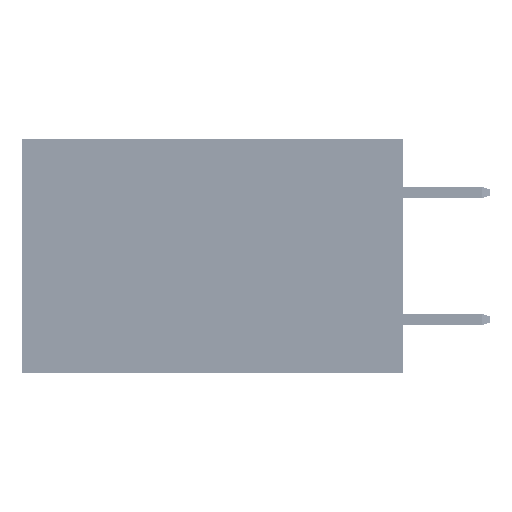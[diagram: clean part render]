
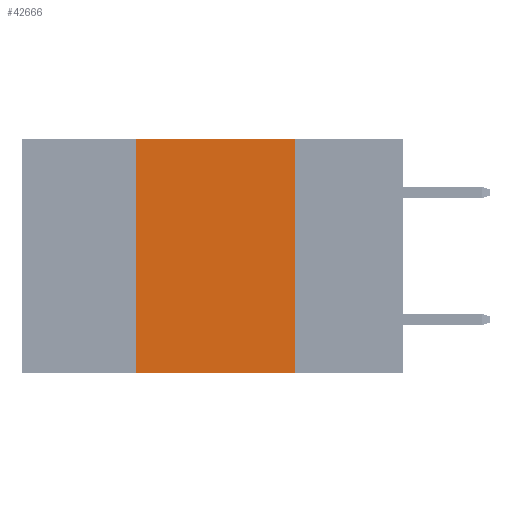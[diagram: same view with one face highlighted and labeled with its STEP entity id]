
A CAD part, left-side view. The second image highlights one B-rep face of the part: STEP entity #42666.
In plain terms, the highlighted planar face has unit normal (-1, 0, 0).
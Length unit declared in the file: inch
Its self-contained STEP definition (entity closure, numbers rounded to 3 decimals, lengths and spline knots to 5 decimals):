
#2341 = DIRECTION ( 'NONE',  ( 1., 0., 0. ) ) ;
#2729 = VERTEX_POINT ( 'NONE', #36102 ) ;
#5283 = CARTESIAN_POINT ( 'NONE',  ( 0., 0.17, -0.37 ) ) ;
#5970 = LINE ( 'NONE', #47476, #14179 ) ;
#6829 = DIRECTION ( 'NONE',  ( 0., -1., 0. ) ) ;
#9076 = DIRECTION ( 'NONE',  ( 0., -1., 0. ) ) ;
#9481 = LINE ( 'NONE', #24145, #21701 ) ;
#11078 = DIRECTION ( 'NONE',  ( 0., 0., 1. ) ) ;
#13001 = CARTESIAN_POINT ( 'NONE',  ( 0., 0.6, 0. ) ) ;
#13865 = VECTOR ( 'NONE', #6829, 39.37008 ) ;
#14179 = VECTOR ( 'NONE', #9076, 39.37008 ) ;
#21701 = VECTOR ( 'NONE', #32241, 39.37008 ) ;
#24145 = CARTESIAN_POINT ( 'NONE',  ( 0., 0.17, 0. ) ) ;
#26279 = CARTESIAN_POINT ( 'NONE',  ( 0., 0.42, 0. ) ) ;
#26647 = EDGE_CURVE ( 'NONE', #44932, #35013, #5970, .T. ) ;
#27323 = VECTOR ( 'NONE', #11078, 39.37008 ) ;
#28458 = PLANE ( 'NONE',  #36567 ) ;
#29786 = VERTEX_POINT ( 'NONE', #30401 ) ;
#30401 = CARTESIAN_POINT ( 'NONE',  ( 0., 0.17, 0. ) ) ;
#32241 = DIRECTION ( 'NONE',  ( 0., 0., -1. ) ) ;
#33123 = LINE ( 'NONE', #26279, #27323 ) ;
#33491 = DIRECTION ( 'NONE',  ( 0., 0., -1. ) ) ;
#34145 = ORIENTED_EDGE ( 'NONE', *, *, #35557, .F. ) ;
#34201 = CARTESIAN_POINT ( 'NONE',  ( 0., 0.6, 0. ) ) ;
#35013 = VERTEX_POINT ( 'NONE', #5283 ) ;
#35150 = EDGE_CURVE ( 'NONE', #2729, #29786, #41501, .T. ) ;
#35557 = EDGE_CURVE ( 'NONE', #44932, #2729, #33123, .T. ) ;
#36102 = CARTESIAN_POINT ( 'NONE',  ( 0., 0.42, 0. ) ) ;
#36290 = FACE_OUTER_BOUND ( 'NONE', #45259, .T. ) ;
#36300 = EDGE_CURVE ( 'NONE', #29786, #35013, #9481, .T. ) ;
#36567 = AXIS2_PLACEMENT_3D ( 'NONE', #13001, #2341, #33491 ) ;
#40978 = ORIENTED_EDGE ( 'NONE', *, *, #35150, .F. ) ;
#41501 = LINE ( 'NONE', #34201, #13865 ) ;
#42666 = ADVANCED_FACE ( 'NONE', ( #36290 ), #28458, .F. ) ;
#44439 = ORIENTED_EDGE ( 'NONE', *, *, #26647, .T. ) ;
#44932 = VERTEX_POINT ( 'NONE', #46752 ) ;
#45259 = EDGE_LOOP ( 'NONE', ( #46855, #40978, #34145, #44439 ) ) ;
#46752 = CARTESIAN_POINT ( 'NONE',  ( 0., 0.42, -0.37 ) ) ;
#46855 = ORIENTED_EDGE ( 'NONE', *, *, #36300, .F. ) ;
#47476 = CARTESIAN_POINT ( 'NONE',  ( 0., 0.6, -0.37 ) ) ;
